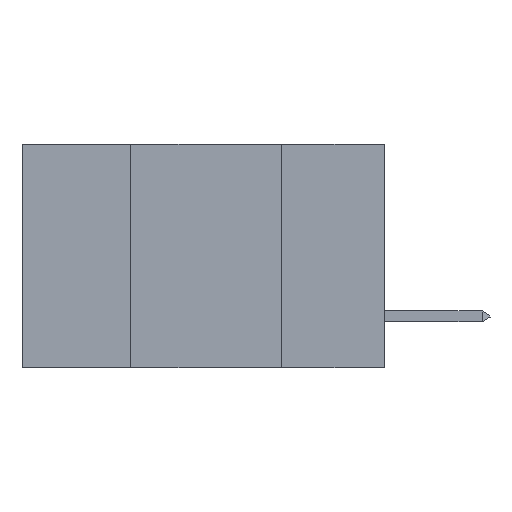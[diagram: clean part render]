
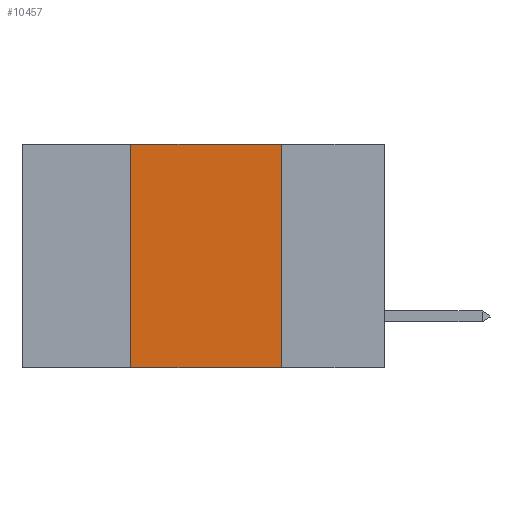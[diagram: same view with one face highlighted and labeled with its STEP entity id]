
A CAD part, left-side view. The second image highlights one B-rep face of the part: STEP entity #10457.
In plain terms, the highlighted planar face has unit normal (-1, 0, 0).
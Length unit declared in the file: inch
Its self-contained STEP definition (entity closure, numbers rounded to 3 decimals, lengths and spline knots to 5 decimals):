
#517 = VERTEX_POINT ( 'NONE', #2866 ) ;
#600 = CARTESIAN_POINT ( 'NONE',  ( 0., 0.17, 0. ) ) ;
#637 = CARTESIAN_POINT ( 'NONE',  ( 0., 0.6, -0.37 ) ) ;
#1312 = VERTEX_POINT ( 'NONE', #2302 ) ;
#1726 = CARTESIAN_POINT ( 'NONE',  ( 0., 0.42, 0. ) ) ;
#1911 = LINE ( 'NONE', #600, #8847 ) ;
#2302 = CARTESIAN_POINT ( 'NONE',  ( 0., 0.42, 0. ) ) ;
#2432 = DIRECTION ( 'NONE',  ( 0., -1., 0. ) ) ;
#2495 = ORIENTED_EDGE ( 'NONE', *, *, #7881, .T. ) ;
#2665 = VECTOR ( 'NONE', #8162, 39.37008 ) ;
#2745 = EDGE_CURVE ( 'NONE', #517, #1312, #9958, .T. ) ;
#2866 = CARTESIAN_POINT ( 'NONE',  ( 0., 0.42, -0.37 ) ) ;
#3117 = VERTEX_POINT ( 'NONE', #3595 ) ;
#3595 = CARTESIAN_POINT ( 'NONE',  ( 0., 0.17, -0.37 ) ) ;
#3714 = FACE_OUTER_BOUND ( 'NONE', #11076, .T. ) ;
#3951 = EDGE_CURVE ( 'NONE', #9916, #3117, #1911, .T. ) ;
#4488 = DIRECTION ( 'NONE',  ( 0., 0., -1. ) ) ;
#4870 = ORIENTED_EDGE ( 'NONE', *, *, #2745, .F. ) ;
#5431 = DIRECTION ( 'NONE',  ( 1., 0., 0. ) ) ;
#5542 = LINE ( 'NONE', #637, #6246 ) ;
#6246 = VECTOR ( 'NONE', #2432, 39.37008 ) ;
#6265 = DIRECTION ( 'NONE',  ( 0., -1., 0. ) ) ;
#6284 = PLANE ( 'NONE',  #8945 ) ;
#6651 = VECTOR ( 'NONE', #6265, 39.37008 ) ;
#6780 = DIRECTION ( 'NONE',  ( 0., 0., -1. ) ) ;
#7194 = ORIENTED_EDGE ( 'NONE', *, *, #8492, .F. ) ;
#7881 = EDGE_CURVE ( 'NONE', #517, #3117, #5542, .T. ) ;
#8014 = CARTESIAN_POINT ( 'NONE',  ( 0., 0.6, 0. ) ) ;
#8162 = DIRECTION ( 'NONE',  ( 0., 0., 1. ) ) ;
#8465 = LINE ( 'NONE', #8891, #6651 ) ;
#8492 = EDGE_CURVE ( 'NONE', #1312, #9916, #8465, .T. ) ;
#8847 = VECTOR ( 'NONE', #6780, 39.37008 ) ;
#8891 = CARTESIAN_POINT ( 'NONE',  ( 0., 0.6, 0. ) ) ;
#8945 = AXIS2_PLACEMENT_3D ( 'NONE', #8014, #5431, #4488 ) ;
#9717 = CARTESIAN_POINT ( 'NONE',  ( 0., 0.17, 0. ) ) ;
#9916 = VERTEX_POINT ( 'NONE', #9717 ) ;
#9958 = LINE ( 'NONE', #1726, #2665 ) ;
#10457 = ADVANCED_FACE ( 'NONE', ( #3714 ), #6284, .F. ) ;
#10901 = ORIENTED_EDGE ( 'NONE', *, *, #3951, .F. ) ;
#11076 = EDGE_LOOP ( 'NONE', ( #10901, #7194, #4870, #2495 ) ) ;
